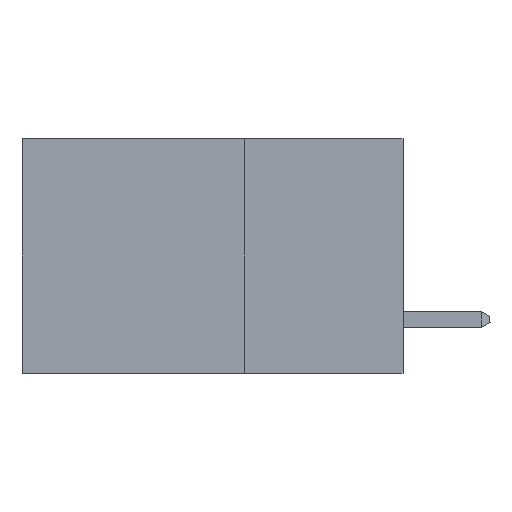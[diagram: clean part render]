
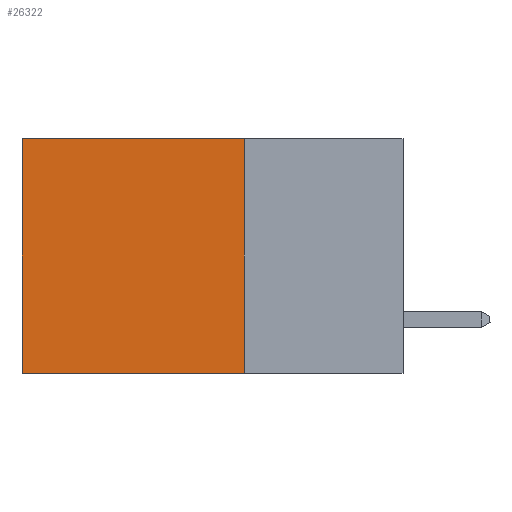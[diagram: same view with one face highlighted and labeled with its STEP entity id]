
A CAD part, left-side view. The second image highlights one B-rep face of the part: STEP entity #26322.
In plain terms, the highlighted planar face has unit normal (-1, 0, 0).
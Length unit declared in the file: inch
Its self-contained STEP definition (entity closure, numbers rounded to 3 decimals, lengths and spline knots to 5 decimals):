
#456 = DIRECTION ( 'NONE',  ( 0., 0., -1. ) ) ;
#505 = CARTESIAN_POINT ( 'NONE',  ( 0.2875, 0.25, 0. ) ) ;
#1101 = CARTESIAN_POINT ( 'NONE',  ( 0.2875, 0.25, 0. ) ) ;
#1842 = LINE ( 'NONE', #505, #24849 ) ;
#1866 = CARTESIAN_POINT ( 'NONE',  ( 0.2875, 0.25, 0. ) ) ;
#4538 = LINE ( 'NONE', #27050, #6194 ) ;
#4701 = VECTOR ( 'NONE', #21700, 39.37008 ) ;
#6194 = VECTOR ( 'NONE', #26953, 39.37008 ) ;
#6329 = LINE ( 'NONE', #11175, #4701 ) ;
#6988 = LINE ( 'NONE', #1866, #8310 ) ;
#7075 = EDGE_CURVE ( 'NONE', #21544, #25682, #6988, .T. ) ;
#8310 = VECTOR ( 'NONE', #456, 39.37008 ) ;
#8616 = ORIENTED_EDGE ( 'NONE', *, *, #20713, .F. ) ;
#10432 = FACE_OUTER_BOUND ( 'NONE', #20520, .T. ) ;
#11175 = CARTESIAN_POINT ( 'NONE',  ( 0.2875, 0.25, -0.37 ) ) ;
#13626 = PLANE ( 'NONE',  #14216 ) ;
#14216 = AXIS2_PLACEMENT_3D ( 'NONE', #1101, #22149, #15938 ) ;
#15185 = ORIENTED_EDGE ( 'NONE', *, *, #26826, .T. ) ;
#15938 = DIRECTION ( 'NONE',  ( 0., 0., -1. ) ) ;
#16110 = VERTEX_POINT ( 'NONE', #24709 ) ;
#17092 = CARTESIAN_POINT ( 'NONE',  ( 0.2875, 0.25, 0. ) ) ;
#17452 = DIRECTION ( 'NONE',  ( 0., 1., 0. ) ) ;
#18619 = ORIENTED_EDGE ( 'NONE', *, *, #7075, .F. ) ;
#19390 = CARTESIAN_POINT ( 'NONE',  ( 0.2875, 0.25, -0.37 ) ) ;
#20520 = EDGE_LOOP ( 'NONE', ( #25807, #8616, #18619, #15185 ) ) ;
#20713 = EDGE_CURVE ( 'NONE', #25682, #23497, #6329, .T. ) ;
#21544 = VERTEX_POINT ( 'NONE', #17092 ) ;
#21700 = DIRECTION ( 'NONE',  ( 0., 1., 0. ) ) ;
#22149 = DIRECTION ( 'NONE',  ( 1., 0., 0. ) ) ;
#23497 = VERTEX_POINT ( 'NONE', #24814 ) ;
#24709 = CARTESIAN_POINT ( 'NONE',  ( 0.2875, 0.6, 0. ) ) ;
#24814 = CARTESIAN_POINT ( 'NONE',  ( 0.2875, 0.6, -0.37 ) ) ;
#24849 = VECTOR ( 'NONE', #17452, 39.37008 ) ;
#25682 = VERTEX_POINT ( 'NONE', #19390 ) ;
#25807 = ORIENTED_EDGE ( 'NONE', *, *, #25898, .T. ) ;
#25898 = EDGE_CURVE ( 'NONE', #16110, #23497, #4538, .T. ) ;
#26322 = ADVANCED_FACE ( 'NONE', ( #10432 ), #13626, .F. ) ;
#26826 = EDGE_CURVE ( 'NONE', #21544, #16110, #1842, .T. ) ;
#26953 = DIRECTION ( 'NONE',  ( 0., 0., -1. ) ) ;
#27050 = CARTESIAN_POINT ( 'NONE',  ( 0.2875, 0.6, 0. ) ) ;
